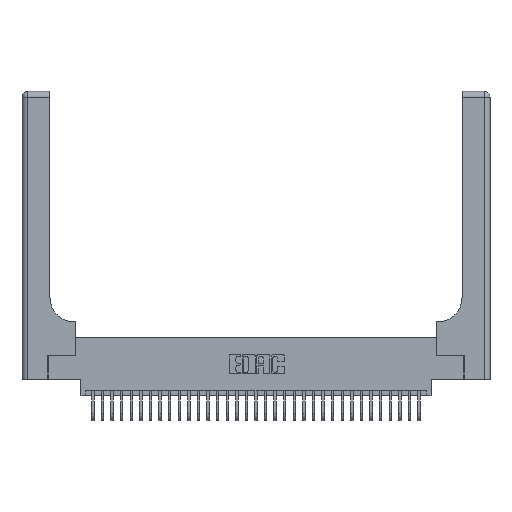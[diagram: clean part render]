
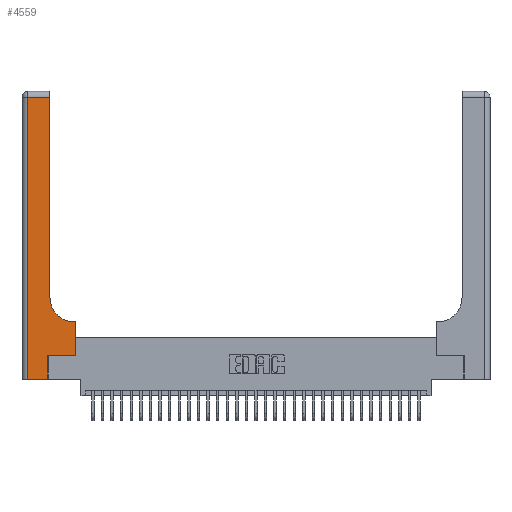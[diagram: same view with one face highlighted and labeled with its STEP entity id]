
A CAD part, top view. The second image highlights one B-rep face of the part: STEP entity #4559.
In plain terms, the highlighted planar face has unit normal (0, 0, 1).
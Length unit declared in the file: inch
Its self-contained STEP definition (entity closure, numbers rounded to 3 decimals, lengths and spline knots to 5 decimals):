
#278 = CARTESIAN_POINT ( 'NONE',  ( 0.2915, 0.85, 0.37 ) ) ;
#471 = LINE ( 'NONE', #26071, #13061 ) ;
#705 = DIRECTION ( 'NONE',  ( -1., 0., 0. ) ) ;
#790 = VERTEX_POINT ( 'NONE', #14339 ) ;
#1028 = VECTOR ( 'NONE', #9788, 39.37008 ) ;
#1259 = VECTOR ( 'NONE', #26432, 39.37008 ) ;
#1280 = LINE ( 'NONE', #7656, #20592 ) ;
#1793 = ORIENTED_EDGE ( 'NONE', *, *, #15878, .T. ) ;
#2023 = LINE ( 'NONE', #15782, #28870 ) ;
#2201 = CARTESIAN_POINT ( 'NONE',  ( 0.06, 2.94, 0.37 ) ) ;
#2249 = LINE ( 'NONE', #11749, #7353 ) ;
#2830 = CARTESIAN_POINT ( 'NONE',  ( 0.06, 0., 0.37 ) ) ;
#3090 = ORIENTED_EDGE ( 'NONE', *, *, #5498, .T. ) ;
#3478 = DIRECTION ( 'NONE',  ( -1., 0., 0. ) ) ;
#4027 = FACE_OUTER_BOUND ( 'NONE', #16480, .T. ) ;
#4222 = ORIENTED_EDGE ( 'NONE', *, *, #9432, .T. ) ;
#4554 = DIRECTION ( 'NONE',  ( -1., 0., 0. ) ) ;
#4559 = ADVANCED_FACE ( 'NONE', ( #4027 ), #13506, .F. ) ;
#4626 = CARTESIAN_POINT ( 'NONE',  ( 0.5585, 0.6, 0.37 ) ) ;
#5498 = EDGE_CURVE ( 'NONE', #20388, #17417, #17033, .T. ) ;
#6133 = LINE ( 'NONE', #14771, #1028 ) ;
#6907 = VECTOR ( 'NONE', #10677, 39.37008 ) ;
#7353 = VECTOR ( 'NONE', #27000, 39.37008 ) ;
#7656 = CARTESIAN_POINT ( 'NONE',  ( 0.2915, 3., 0.37 ) ) ;
#9432 = EDGE_CURVE ( 'NONE', #17417, #20147, #1280, .T. ) ;
#9788 = DIRECTION ( 'NONE',  ( 1., 0., 0. ) ) ;
#9895 = AXIS2_PLACEMENT_3D ( 'NONE', #16042, #18551, #3478 ) ;
#10557 = ORIENTED_EDGE ( 'NONE', *, *, #31420, .T. ) ;
#10677 = DIRECTION ( 'NONE',  ( 0., -1., 0. ) ) ;
#11316 = CARTESIAN_POINT ( 'NONE',  ( 0., 0., 0.37 ) ) ;
#11595 = CARTESIAN_POINT ( 'NONE',  ( 0.5415, 0.85, 0.37 ) ) ;
#11749 = CARTESIAN_POINT ( 'NONE',  ( 0.269, 0., 0.37 ) ) ;
#12408 = VECTOR ( 'NONE', #4554, 39.37008 ) ;
#13029 = ORIENTED_EDGE ( 'NONE', *, *, #29201, .T. ) ;
#13061 = VECTOR ( 'NONE', #18530, 39.37008 ) ;
#13506 = PLANE ( 'NONE',  #9895 ) ;
#14118 = DIRECTION ( 'NONE',  ( 1., 0., 0. ) ) ;
#14319 = CARTESIAN_POINT ( 'NONE',  ( 0.269, 0.25, 0.37 ) ) ;
#14339 = CARTESIAN_POINT ( 'NONE',  ( 0.269, 0., 0.37 ) ) ;
#14771 = CARTESIAN_POINT ( 'NONE',  ( 0.269, 0.25, 0.37 ) ) ;
#14784 = LINE ( 'NONE', #29824, #12408 ) ;
#15782 = CARTESIAN_POINT ( 'NONE',  ( 0.2915, 0.6, 0.37 ) ) ;
#15796 = CARTESIAN_POINT ( 'NONE',  ( 0.5585, 0.25, 0.37 ) ) ;
#15878 = EDGE_CURVE ( 'NONE', #30069, #24480, #19527, .T. ) ;
#16042 = CARTESIAN_POINT ( 'NONE',  ( 0., 3., 0.37 ) ) ;
#16480 = EDGE_LOOP ( 'NONE', ( #4222, #30936, #1793, #28021, #10557, #31333, #13029, #20211, #3090 ) ) ;
#16693 = VERTEX_POINT ( 'NONE', #4626 ) ;
#17033 = CIRCLE ( 'NONE', #30645, 0.25 ) ;
#17417 = VERTEX_POINT ( 'NONE', #278 ) ;
#18271 = CARTESIAN_POINT ( 'NONE',  ( 0.06, 3., 0.37 ) ) ;
#18440 = VERTEX_POINT ( 'NONE', #14319 ) ;
#18530 = DIRECTION ( 'NONE',  ( 0., 1., 0. ) ) ;
#18551 = DIRECTION ( 'NONE',  ( 0., 0., -1. ) ) ;
#19527 = LINE ( 'NONE', #18271, #6907 ) ;
#19757 = EDGE_CURVE ( 'NONE', #18440, #29123, #6133, .T. ) ;
#20147 = VERTEX_POINT ( 'NONE', #26450 ) ;
#20211 = ORIENTED_EDGE ( 'NONE', *, *, #23197, .T. ) ;
#20388 = VERTEX_POINT ( 'NONE', #24668 ) ;
#20592 = VECTOR ( 'NONE', #27877, 39.37008 ) ;
#21058 = EDGE_CURVE ( 'NONE', #20147, #30069, #14784, .T. ) ;
#21378 = LINE ( 'NONE', #11316, #1259 ) ;
#22729 = EDGE_CURVE ( 'NONE', #24480, #790, #21378, .T. ) ;
#23197 = EDGE_CURVE ( 'NONE', #16693, #20388, #2023, .T. ) ;
#24480 = VERTEX_POINT ( 'NONE', #2830 ) ;
#24668 = CARTESIAN_POINT ( 'NONE',  ( 0.5415, 0.6, 0.37 ) ) ;
#26071 = CARTESIAN_POINT ( 'NONE',  ( 0.5585, 0.25, 0.37 ) ) ;
#26432 = DIRECTION ( 'NONE',  ( 1., 0., 0. ) ) ;
#26450 = CARTESIAN_POINT ( 'NONE',  ( 0.2915, 2.94, 0.37 ) ) ;
#27000 = DIRECTION ( 'NONE',  ( 0., 1., 0. ) ) ;
#27877 = DIRECTION ( 'NONE',  ( 0., 1., 0. ) ) ;
#28021 = ORIENTED_EDGE ( 'NONE', *, *, #22729, .T. ) ;
#28870 = VECTOR ( 'NONE', #705, 39.37008 ) ;
#29123 = VERTEX_POINT ( 'NONE', #15796 ) ;
#29201 = EDGE_CURVE ( 'NONE', #29123, #16693, #471, .T. ) ;
#29261 = DIRECTION ( 'NONE',  ( 0., 0., -1. ) ) ;
#29824 = CARTESIAN_POINT ( 'NONE',  ( 0., 2.94, 0.37 ) ) ;
#30069 = VERTEX_POINT ( 'NONE', #2201 ) ;
#30645 = AXIS2_PLACEMENT_3D ( 'NONE', #11595, #29261, #14118 ) ;
#30936 = ORIENTED_EDGE ( 'NONE', *, *, #21058, .T. ) ;
#31333 = ORIENTED_EDGE ( 'NONE', *, *, #19757, .T. ) ;
#31420 = EDGE_CURVE ( 'NONE', #790, #18440, #2249, .T. ) ;
